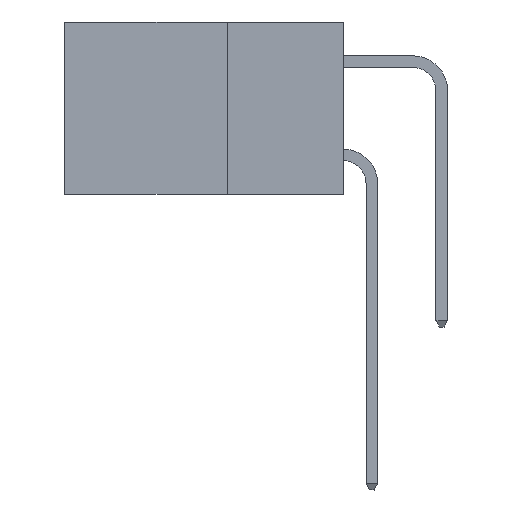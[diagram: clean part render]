
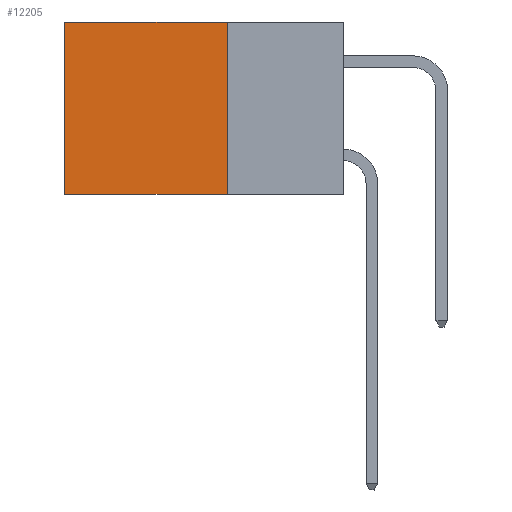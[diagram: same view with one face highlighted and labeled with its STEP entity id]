
A CAD part, left-side view. The second image highlights one B-rep face of the part: STEP entity #12205.
In plain terms, the highlighted planar face has unit normal (-1, 0, 0).
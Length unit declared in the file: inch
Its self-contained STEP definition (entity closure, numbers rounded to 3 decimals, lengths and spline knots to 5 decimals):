
#152 = ORIENTED_EDGE ( 'NONE', *, *, #13830, .T. ) ;
#358 = DIRECTION ( 'NONE',  ( 0., 0., -1. ) ) ;
#449 = EDGE_LOOP ( 'NONE', ( #152, #2350, #27398, #15456 ) ) ;
#578 = CARTESIAN_POINT ( 'NONE',  ( 0.298, 0.25, 0. ) ) ;
#609 = LINE ( 'NONE', #6379, #2315 ) ;
#1030 = VERTEX_POINT ( 'NONE', #1199 ) ;
#1199 = CARTESIAN_POINT ( 'NONE',  ( 0.298, 0.25, -0.37 ) ) ;
#2315 = VECTOR ( 'NONE', #27516, 39.37008 ) ;
#2350 = ORIENTED_EDGE ( 'NONE', *, *, #10484, .F. ) ;
#2491 = VERTEX_POINT ( 'NONE', #27381 ) ;
#4166 = EDGE_CURVE ( 'NONE', #27556, #8923, #17563, .T. ) ;
#6379 = CARTESIAN_POINT ( 'NONE',  ( 0.298, 0.25, 0. ) ) ;
#6744 = CARTESIAN_POINT ( 'NONE',  ( 0.298, 0.25, 0. ) ) ;
#6946 = DIRECTION ( 'NONE',  ( 0., 1., 0. ) ) ;
#8923 = VERTEX_POINT ( 'NONE', #25772 ) ;
#8925 = DIRECTION ( 'NONE',  ( 0., 1., 0. ) ) ;
#10206 = CARTESIAN_POINT ( 'NONE',  ( 0.298, 0.6, 0. ) ) ;
#10484 = EDGE_CURVE ( 'NONE', #1030, #2491, #13598, .T. ) ;
#11342 = CARTESIAN_POINT ( 'NONE',  ( 0.298, 0.25, -0.37 ) ) ;
#12205 = ADVANCED_FACE ( 'NONE', ( #26341 ), #17455, .F. ) ;
#13598 = LINE ( 'NONE', #11342, #18973 ) ;
#13830 = EDGE_CURVE ( 'NONE', #8923, #2491, #21463, .T. ) ;
#15290 = DIRECTION ( 'NONE',  ( 1., 0., 0. ) ) ;
#15456 = ORIENTED_EDGE ( 'NONE', *, *, #4166, .T. ) ;
#17455 = PLANE ( 'NONE',  #26212 ) ;
#17563 = LINE ( 'NONE', #578, #27026 ) ;
#18973 = VECTOR ( 'NONE', #6946, 39.37008 ) ;
#19150 = VECTOR ( 'NONE', #23412, 39.37008 ) ;
#21463 = LINE ( 'NONE', #10206, #19150 ) ;
#22382 = EDGE_CURVE ( 'NONE', #27556, #1030, #609, .T. ) ;
#23412 = DIRECTION ( 'NONE',  ( 0., 0., -1. ) ) ;
#24612 = CARTESIAN_POINT ( 'NONE',  ( 0.298, 0.25, 0. ) ) ;
#25772 = CARTESIAN_POINT ( 'NONE',  ( 0.298, 0.6, 0. ) ) ;
#26212 = AXIS2_PLACEMENT_3D ( 'NONE', #6744, #15290, #358 ) ;
#26341 = FACE_OUTER_BOUND ( 'NONE', #449, .T. ) ;
#27026 = VECTOR ( 'NONE', #8925, 39.37008 ) ;
#27381 = CARTESIAN_POINT ( 'NONE',  ( 0.298, 0.6, -0.37 ) ) ;
#27398 = ORIENTED_EDGE ( 'NONE', *, *, #22382, .F. ) ;
#27516 = DIRECTION ( 'NONE',  ( 0., 0., -1. ) ) ;
#27556 = VERTEX_POINT ( 'NONE', #24612 ) ;
